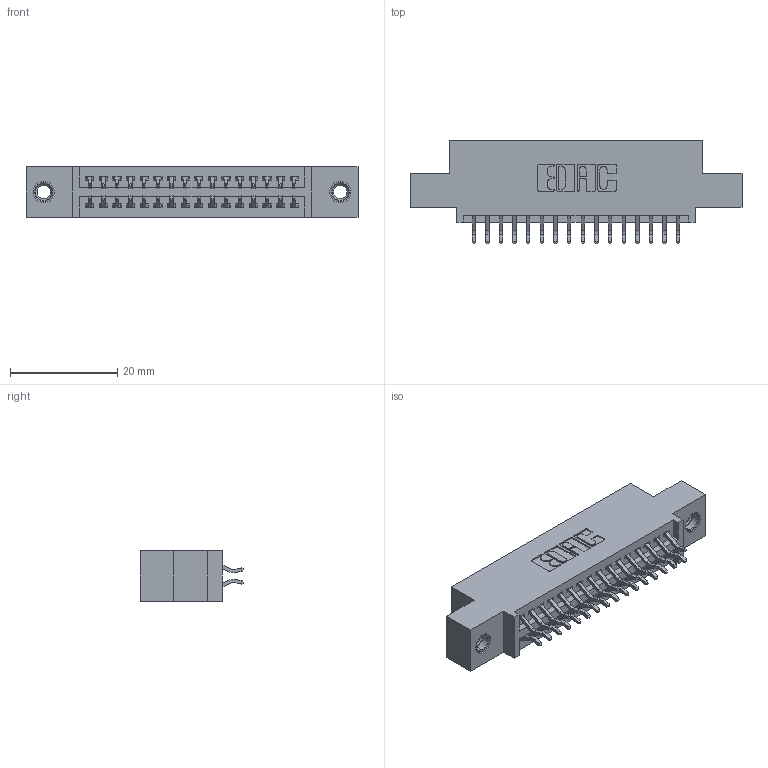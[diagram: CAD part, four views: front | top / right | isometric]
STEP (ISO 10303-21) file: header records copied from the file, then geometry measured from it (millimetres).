
FILE_DESCRIPTION (( 'STEP AP203' ), '1' );
FILE_NAME ('395-032-556-507.STEP', '2018-11-12T22:48:33', ( '' ), ( '' ), 'SwSTEP 2.0', 'SolidWorks 2016', '' );
FILE_SCHEMA (( 'CONFIG_CONTROL_DESIGN' ));
Length unit declared in the file: inch
Products named in the file (4): 395-032-556-507; 345-250-001_345-250-005-103; 345 Part_0.110 Offset - 0.156 Dia-TI; 345-292-001_556 Tail
Assembly tree (35 placements, depth 2):
  395-032-556-507
    345 Part_0.110 Offset - 0.156 Dia-TI
    345-292-001_556 Tail  x32
    345-250-001_345-250-005-103  x2
Bounding box: 61.85 x 19.24 x 9.4 mm (x, y, z)
Volume: 5678.6 mm3; surface area: 7983 mm2
Topology: 35 solids, 35 shells, 1982 faces, 5833 edges, 3838 vertices
Faces by surface type: plane 1300, cylinder 666, cone 12, torus 4
Entity records: 17592 total; most frequent: CARTESIAN_POINT 2971, ORIENTED_EDGE 2886, DIRECTION 2665, EDGE_CURVE 1443, VECTOR 1219, LINE 1219, VERTEX_POINT 956, AXIS2_PLACEMENT_3D 723
